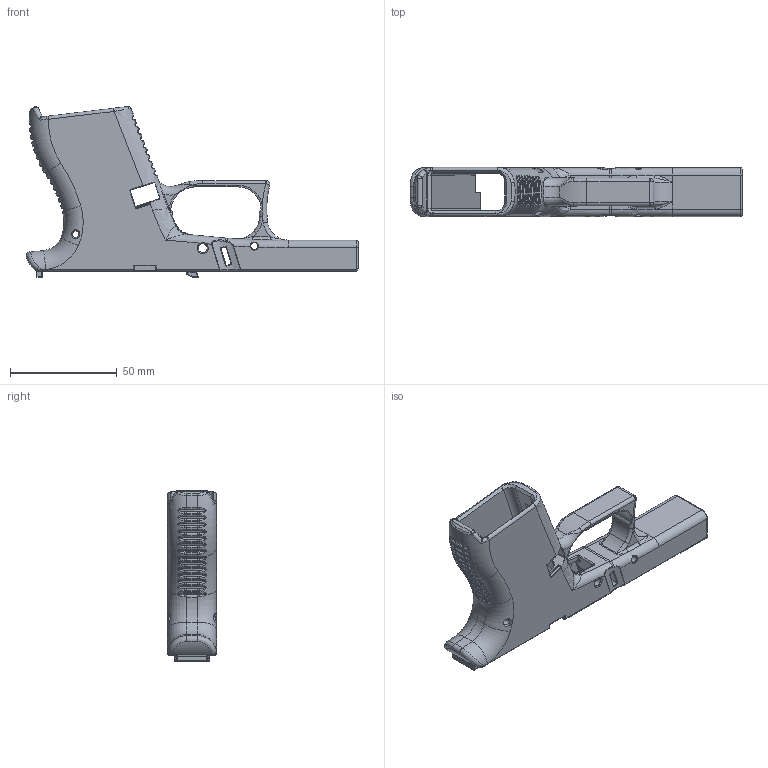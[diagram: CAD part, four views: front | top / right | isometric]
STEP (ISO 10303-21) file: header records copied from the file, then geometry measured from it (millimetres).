
FILE_DESCRIPTION(/* description */ (''),/* implementation_level */ '2;1');
FILE_NAME(/* name */ 'Frame.step',/* time_stamp */ '2021-09-17T03:43:16-04:00',/* author */ (''),/* organization */ (''),/* preprocessor_version */ 'ST-DEVELOPER v18.1',/* originating_system */ 'Autodesk Translation Framework v10.10.0.1391',/* authorisation */ '');
FILE_SCHEMA (('AUTOMOTIVE_DESIGN { 1 0 10303 214 3 1 1 }'));
Products named in the file (2): Frame; Rails and Internals
Assembly tree (1 placements, depth 2):
  Frame
    Rails and Internals
Bounding box: 155.83 x 23 x 80.21 mm (x, y, z)
Volume: 48734.6 mm3; surface area: 32094.3 mm2
Topology: 1 solids, 1 shells, 1308 faces, 3276 edges, 1903 vertices
Faces by surface type: bspline 526, cylinder 397, plane 231, torus 103, sphere 29, cone 22
Full cylindrical faces by diameter (mm): 3.05 x2, 3.3 x2, 3.5 x1, 4.25 x2
Entity records: 55783 total; most frequent: CARTESIAN_POINT 26612, ORIENTED_EDGE 6454, DIRECTION 5715, EDGE_CURVE 3227, AXIS2_PLACEMENT_3D 2333, VERTEX_POINT 1903, EDGE_LOOP 1316, FACE_OUTER_BOUND 1308
